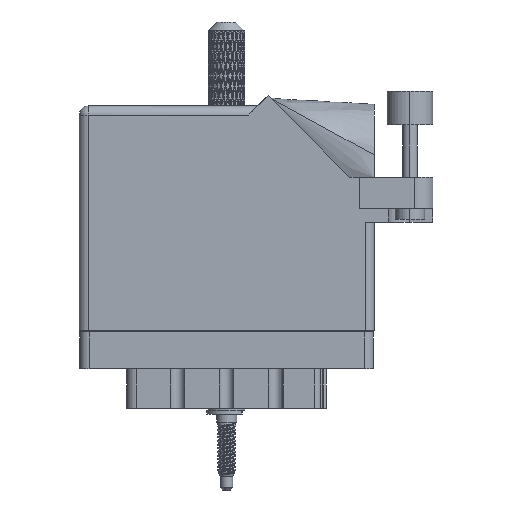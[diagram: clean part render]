
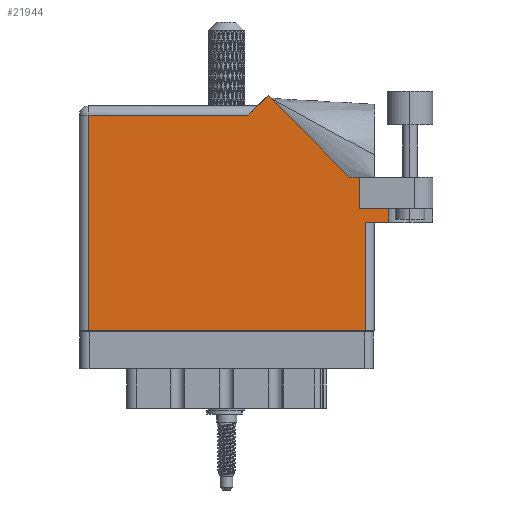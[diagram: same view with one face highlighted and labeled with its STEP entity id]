
A CAD part, front view. The second image highlights one B-rep face of the part: STEP entity #21944.
In plain terms, the highlighted face is planar.
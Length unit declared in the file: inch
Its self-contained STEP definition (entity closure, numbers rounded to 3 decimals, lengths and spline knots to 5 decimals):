
#1040 = DIRECTION ( 'NONE',  ( 1., 0., 0. ) ) ;
#3168 = LINE ( 'NONE', #50488, #59211 ) ;
#6490 = CARTESIAN_POINT ( 'NONE',  ( 1.948, 0., 0. ) ) ;
#8860 = LINE ( 'NONE', #82191, #44261 ) ;
#9768 = ORIENTED_EDGE ( 'NONE', *, *, #18818, .T. ) ;
#10390 = EDGE_CURVE ( 'NONE', #97950, #21995, #62261, .T. ) ;
#13307 = VECTOR ( 'NONE', #46385, 39.37008 ) ;
#15025 = VECTOR ( 'NONE', #84285, 39.37008 ) ;
#17149 = ORIENTED_EDGE ( 'NONE', *, *, #91239, .T. ) ;
#18402 = CARTESIAN_POINT ( 'NONE',  ( 1.91, 0.831, 0. ) ) ;
#18818 = EDGE_CURVE ( 'NONE', #73357, #71603, #104676, .T. ) ;
#21115 = CARTESIAN_POINT ( 'NONE',  ( 1.217, 1.53, 0. ) ) ;
#21944 = ADVANCED_FACE ( 'NONE', ( #78916 ), #32733, .F. ) ;
#21995 = VERTEX_POINT ( 'NONE', #48495 ) ;
#23642 = LINE ( 'NONE', #56194, #43654 ) ;
#23674 = VERTEX_POINT ( 'NONE', #93438 ) ;
#23683 = VECTOR ( 'NONE', #65884, 39.37008 ) ;
#23872 = DIRECTION ( 'NONE',  ( 1., 0., 0. ) ) ;
#24645 = CARTESIAN_POINT ( 'NONE',  ( 2.1115, 0.831, 0. ) ) ;
#26932 = DIRECTION ( 'NONE',  ( -1., 0., 0. ) ) ;
#27058 = VERTEX_POINT ( 'NONE', #24645 ) ;
#28375 = VECTOR ( 'NONE', #23872, 39.37008 ) ;
#28905 = VECTOR ( 'NONE', #86106, 39.37008 ) ;
#31122 = DIRECTION ( 'NONE',  ( 0., 0., -1. ) ) ;
#31235 = CARTESIAN_POINT ( 'NONE',  ( 1.28771, 1.60071, 0. ) ) ;
#32733 = PLANE ( 'NONE',  #84500 ) ;
#34074 = EDGE_CURVE ( 'NONE', #34890, #41512, #66637, .T. ) ;
#34890 = VERTEX_POINT ( 'NONE', #66471 ) ;
#35035 = ORIENTED_EDGE ( 'NONE', *, *, #104174, .T. ) ;
#38293 = VECTOR ( 'NONE', #40060, 39.37008 ) ;
#38745 = ORIENTED_EDGE ( 'NONE', *, *, #50014, .T. ) ;
#38884 = VERTEX_POINT ( 'NONE', #69523 ) ;
#40060 = DIRECTION ( 'NONE',  ( 0., -1., 0. ) ) ;
#41155 = DIRECTION ( 'NONE',  ( -0.707, -0.707, 0. ) ) ;
#41236 = ORIENTED_EDGE ( 'NONE', *, *, #56801, .T. ) ;
#41512 = VERTEX_POINT ( 'NONE', #75007 ) ;
#41995 = VERTEX_POINT ( 'NONE', #18402 ) ;
#43654 = VECTOR ( 'NONE', #96370, 39.37008 ) ;
#44261 = VECTOR ( 'NONE', #98481, 39.37008 ) ;
#44289 = CARTESIAN_POINT ( 'NONE',  ( 2.41, 1.044, 0. ) ) ;
#44941 = EDGE_CURVE ( 'NONE', #27058, #64375, #23642, .T. ) ;
#46385 = DIRECTION ( 'NONE',  ( -0.707, 0.707, 0. ) ) ;
#48495 = CARTESIAN_POINT ( 'NONE',  ( 1.948, 0.737, 0. ) ) ;
#50014 = EDGE_CURVE ( 'NONE', #23674, #38884, #84993, .T. ) ;
#50488 = CARTESIAN_POINT ( 'NONE',  ( 1.91, 0.831, 0. ) ) ;
#54335 = CARTESIAN_POINT ( 'NONE',  ( 1.155, 1.468, 0. ) ) ;
#56194 = CARTESIAN_POINT ( 'NONE',  ( 2.1115, 1.16177, 0. ) ) ;
#56801 = EDGE_CURVE ( 'NONE', #41995, #23674, #8860, .T. ) ;
#57164 = CARTESIAN_POINT ( 'NONE',  ( 0., 1.53, 0. ) ) ;
#59211 = VECTOR ( 'NONE', #1040, 39.37008 ) ;
#60189 = EDGE_CURVE ( 'NONE', #38884, #73357, #70255, .T. ) ;
#60278 = EDGE_CURVE ( 'NONE', #71603, #34890, #82143, .T. ) ;
#60931 = CARTESIAN_POINT ( 'NONE',  ( 0., 0., 0. ) ) ;
#62261 = LINE ( 'NONE', #87178, #28905 ) ;
#64375 = VERTEX_POINT ( 'NONE', #94411 ) ;
#64763 = DIRECTION ( 'NONE',  ( -1., 0., 0. ) ) ;
#65255 = VECTOR ( 'NONE', #41155, 39.37008 ) ;
#65589 = CARTESIAN_POINT ( 'NONE',  ( 0.062, 0., 0. ) ) ;
#65884 = DIRECTION ( 'NONE',  ( -1., 0., 0. ) ) ;
#66471 = CARTESIAN_POINT ( 'NONE',  ( 0.062, 1.468, 0. ) ) ;
#66637 = LINE ( 'NONE', #65589, #38293 ) ;
#69523 = CARTESIAN_POINT ( 'NONE',  ( 1.84442, 1.044, 0. ) ) ;
#70148 = LINE ( 'NONE', #60931, #15025 ) ;
#70255 = LINE ( 'NONE', #71864, #13307 ) ;
#71603 = VERTEX_POINT ( 'NONE', #54335 ) ;
#71864 = CARTESIAN_POINT ( 'NONE',  ( 1.84442, 1.044, 0. ) ) ;
#73357 = VERTEX_POINT ( 'NONE', #31235 ) ;
#75007 = CARTESIAN_POINT ( 'NONE',  ( 0.062, 0., 0. ) ) ;
#76153 = EDGE_CURVE ( 'NONE', #41995, #27058, #3168, .T. ) ;
#77563 = EDGE_LOOP ( 'NONE', ( #17149, #88510, #35035, #105561, #80427, #41236, #38745, #103668, #9768, #99290, #79639 ) ) ;
#78916 = FACE_OUTER_BOUND ( 'NONE', #77563, .T. ) ;
#79639 = ORIENTED_EDGE ( 'NONE', *, *, #34074, .T. ) ;
#80427 = ORIENTED_EDGE ( 'NONE', *, *, #76153, .F. ) ;
#82143 = LINE ( 'NONE', #91349, #23683 ) ;
#82191 = CARTESIAN_POINT ( 'NONE',  ( 1.91, 0.831, 0. ) ) ;
#82467 = CARTESIAN_POINT ( 'NONE',  ( 2.01, 0.737, 0. ) ) ;
#84285 = DIRECTION ( 'NONE',  ( 1., 0., 0. ) ) ;
#84500 = AXIS2_PLACEMENT_3D ( 'NONE', #57164, #31122, #64763 ) ;
#84993 = LINE ( 'NONE', #44289, #90525 ) ;
#86106 = DIRECTION ( 'NONE',  ( 0., 1., 0. ) ) ;
#87178 = CARTESIAN_POINT ( 'NONE',  ( 1.948, 0.737, 0. ) ) ;
#88510 = ORIENTED_EDGE ( 'NONE', *, *, #10390, .T. ) ;
#90525 = VECTOR ( 'NONE', #26932, 39.37008 ) ;
#91239 = EDGE_CURVE ( 'NONE', #41512, #97950, #70148, .T. ) ;
#91349 = CARTESIAN_POINT ( 'NONE',  ( 0., 1.468, 0. ) ) ;
#91672 = LINE ( 'NONE', #82467, #28375 ) ;
#93438 = CARTESIAN_POINT ( 'NONE',  ( 1.91, 1.044, 0. ) ) ;
#94411 = CARTESIAN_POINT ( 'NONE',  ( 2.1115, 0.737, 0. ) ) ;
#96370 = DIRECTION ( 'NONE',  ( 0., -1., 0. ) ) ;
#97950 = VERTEX_POINT ( 'NONE', #6490 ) ;
#98481 = DIRECTION ( 'NONE',  ( 0., 1., 0. ) ) ;
#99290 = ORIENTED_EDGE ( 'NONE', *, *, #60278, .T. ) ;
#103668 = ORIENTED_EDGE ( 'NONE', *, *, #60189, .T. ) ;
#104174 = EDGE_CURVE ( 'NONE', #21995, #64375, #91672, .T. ) ;
#104676 = LINE ( 'NONE', #21115, #65255 ) ;
#105561 = ORIENTED_EDGE ( 'NONE', *, *, #44941, .F. ) ;
